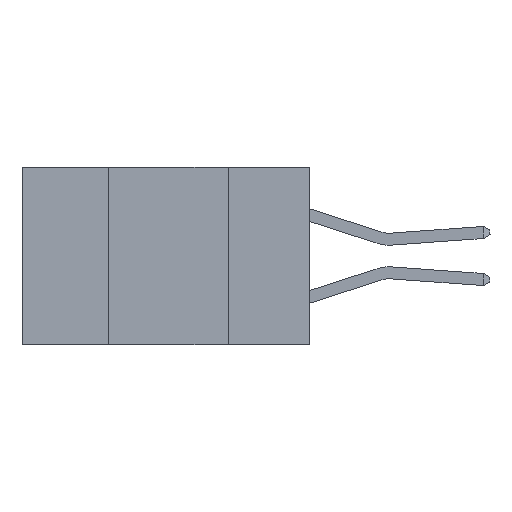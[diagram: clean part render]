
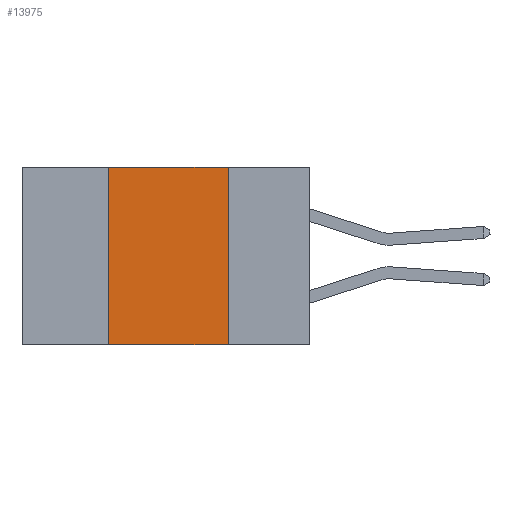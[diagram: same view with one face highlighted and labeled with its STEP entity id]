
A CAD part, left-side view. The second image highlights one B-rep face of the part: STEP entity #13975.
In plain terms, the highlighted planar face has unit normal (-1, 0, 0).
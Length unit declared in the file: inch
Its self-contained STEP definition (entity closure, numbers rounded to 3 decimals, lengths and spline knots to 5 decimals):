
#24 = ORIENTED_EDGE ( 'NONE', *, *, #5405, .T. ) ;
#124 = VERTEX_POINT ( 'NONE', #8782 ) ;
#790 = VECTOR ( 'NONE', #12545, 39.37008 ) ;
#1263 = LINE ( 'NONE', #4475, #13159 ) ;
#1530 = EDGE_LOOP ( 'NONE', ( #13912, #6684, #7896, #24 ) ) ;
#1556 = VERTEX_POINT ( 'NONE', #5733 ) ;
#1566 = AXIS2_PLACEMENT_3D ( 'NONE', #3989, #11735, #5265 ) ;
#1695 = CARTESIAN_POINT ( 'NONE',  ( 0., 0.6, 0. ) ) ;
#1767 = PLANE ( 'NONE',  #1566 ) ;
#2155 = VECTOR ( 'NONE', #10380, 39.37008 ) ;
#2566 = EDGE_CURVE ( 'NONE', #13708, #1556, #6668, .T. ) ;
#3076 = EDGE_CURVE ( 'NONE', #124, #13708, #6045, .T. ) ;
#3989 = CARTESIAN_POINT ( 'NONE',  ( 0., 0.6, 0. ) ) ;
#4475 = CARTESIAN_POINT ( 'NONE',  ( 0., 0.42, -0.37 ) ) ;
#4525 = CARTESIAN_POINT ( 'NONE',  ( 0., 0.17, -0.37 ) ) ;
#4853 = VERTEX_POINT ( 'NONE', #5549 ) ;
#5265 = DIRECTION ( 'NONE',  ( 0., 0., -1. ) ) ;
#5405 = EDGE_CURVE ( 'NONE', #4853, #1556, #11421, .T. ) ;
#5549 = CARTESIAN_POINT ( 'NONE',  ( 0., 0.42, -0.37 ) ) ;
#5733 = CARTESIAN_POINT ( 'NONE',  ( 0., 0.17, -0.37 ) ) ;
#6045 = LINE ( 'NONE', #1695, #2155 ) ;
#6668 = LINE ( 'NONE', #4525, #10316 ) ;
#6684 = ORIENTED_EDGE ( 'NONE', *, *, #3076, .F. ) ;
#7896 = ORIENTED_EDGE ( 'NONE', *, *, #14011, .F. ) ;
#8216 = CARTESIAN_POINT ( 'NONE',  ( 0., 0.6, -0.37 ) ) ;
#8541 = DIRECTION ( 'NONE',  ( 0., 0., 1. ) ) ;
#8782 = CARTESIAN_POINT ( 'NONE',  ( 0., 0.42, 0. ) ) ;
#8877 = DIRECTION ( 'NONE',  ( 0., 0., -1. ) ) ;
#9248 = CARTESIAN_POINT ( 'NONE',  ( 0., 0.17, 0. ) ) ;
#10316 = VECTOR ( 'NONE', #8877, 39.37008 ) ;
#10380 = DIRECTION ( 'NONE',  ( 0., -1., 0. ) ) ;
#11421 = LINE ( 'NONE', #8216, #790 ) ;
#11592 = FACE_OUTER_BOUND ( 'NONE', #1530, .T. ) ;
#11735 = DIRECTION ( 'NONE',  ( 1., 0., 0. ) ) ;
#12545 = DIRECTION ( 'NONE',  ( 0., -1., 0. ) ) ;
#13159 = VECTOR ( 'NONE', #8541, 39.37008 ) ;
#13708 = VERTEX_POINT ( 'NONE', #9248 ) ;
#13912 = ORIENTED_EDGE ( 'NONE', *, *, #2566, .F. ) ;
#13975 = ADVANCED_FACE ( 'NONE', ( #11592 ), #1767, .F. ) ;
#14011 = EDGE_CURVE ( 'NONE', #4853, #124, #1263, .T. ) ;
